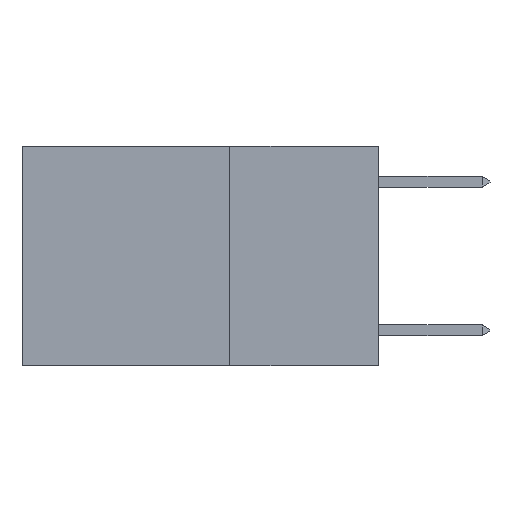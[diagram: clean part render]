
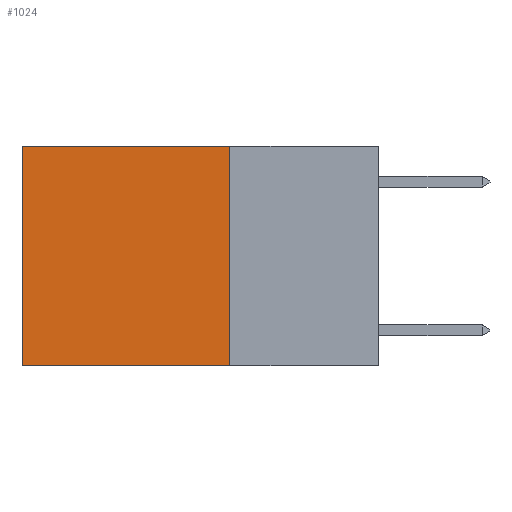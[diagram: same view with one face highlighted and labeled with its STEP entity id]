
A CAD part, left-side view. The second image highlights one B-rep face of the part: STEP entity #1024.
In plain terms, the highlighted planar face has unit normal (-1, 0, 0).
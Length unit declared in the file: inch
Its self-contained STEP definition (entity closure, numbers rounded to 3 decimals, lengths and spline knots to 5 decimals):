
#555 = EDGE_CURVE ( 'NONE', #8140, #2084, #6024, .T. ) ;
#609 = DIRECTION ( 'NONE',  ( 0., 0., -1. ) ) ;
#748 = DIRECTION ( 'NONE',  ( 1., 0., 0. ) ) ;
#833 = CARTESIAN_POINT ( 'NONE',  ( 0.2625, 0.25, 0. ) ) ;
#839 = VERTEX_POINT ( 'NONE', #11322 ) ;
#1024 = ADVANCED_FACE ( 'NONE', ( #11215 ), #1120, .F. ) ;
#1120 = PLANE ( 'NONE',  #11615 ) ;
#1887 = EDGE_CURVE ( 'NONE', #12315, #839, #6559, .T. ) ;
#2084 = VERTEX_POINT ( 'NONE', #3655 ) ;
#2394 = EDGE_LOOP ( 'NONE', ( #5607, #3464, #10810, #3756 ) ) ;
#2717 = CARTESIAN_POINT ( 'NONE',  ( 0.2625, 0.6, 0. ) ) ;
#3464 = ORIENTED_EDGE ( 'NONE', *, *, #1887, .F. ) ;
#3655 = CARTESIAN_POINT ( 'NONE',  ( 0.2625, 0.6, 0. ) ) ;
#3756 = ORIENTED_EDGE ( 'NONE', *, *, #555, .T. ) ;
#4928 = DIRECTION ( 'NONE',  ( 0., 0., -1. ) ) ;
#5607 = ORIENTED_EDGE ( 'NONE', *, *, #8348, .T. ) ;
#5776 = DIRECTION ( 'NONE',  ( 0., 1., 0. ) ) ;
#6024 = LINE ( 'NONE', #9234, #8148 ) ;
#6274 = CARTESIAN_POINT ( 'NONE',  ( 0.2625, 0.25, 0. ) ) ;
#6559 = LINE ( 'NONE', #12285, #11190 ) ;
#6604 = VECTOR ( 'NONE', #11072, 39.37008 ) ;
#6738 = CARTESIAN_POINT ( 'NONE',  ( 0.2625, 0.25, 0. ) ) ;
#7169 = LINE ( 'NONE', #2717, #6604 ) ;
#7910 = DIRECTION ( 'NONE',  ( 0., 1., 0. ) ) ;
#8067 = VECTOR ( 'NONE', #4928, 39.37008 ) ;
#8140 = VERTEX_POINT ( 'NONE', #6274 ) ;
#8148 = VECTOR ( 'NONE', #7910, 39.37008 ) ;
#8348 = EDGE_CURVE ( 'NONE', #2084, #839, #7169, .T. ) ;
#9161 = CARTESIAN_POINT ( 'NONE',  ( 0.2625, 0.25, -0.37 ) ) ;
#9234 = CARTESIAN_POINT ( 'NONE',  ( 0.2625, 0.25, 0. ) ) ;
#9775 = EDGE_CURVE ( 'NONE', #8140, #12315, #10566, .T. ) ;
#10566 = LINE ( 'NONE', #6738, #8067 ) ;
#10810 = ORIENTED_EDGE ( 'NONE', *, *, #9775, .F. ) ;
#11072 = DIRECTION ( 'NONE',  ( 0., 0., -1. ) ) ;
#11190 = VECTOR ( 'NONE', #5776, 39.37008 ) ;
#11215 = FACE_OUTER_BOUND ( 'NONE', #2394, .T. ) ;
#11322 = CARTESIAN_POINT ( 'NONE',  ( 0.2625, 0.6, -0.37 ) ) ;
#11615 = AXIS2_PLACEMENT_3D ( 'NONE', #833, #748, #609 ) ;
#12285 = CARTESIAN_POINT ( 'NONE',  ( 0.2625, 0.25, -0.37 ) ) ;
#12315 = VERTEX_POINT ( 'NONE', #9161 ) ;
